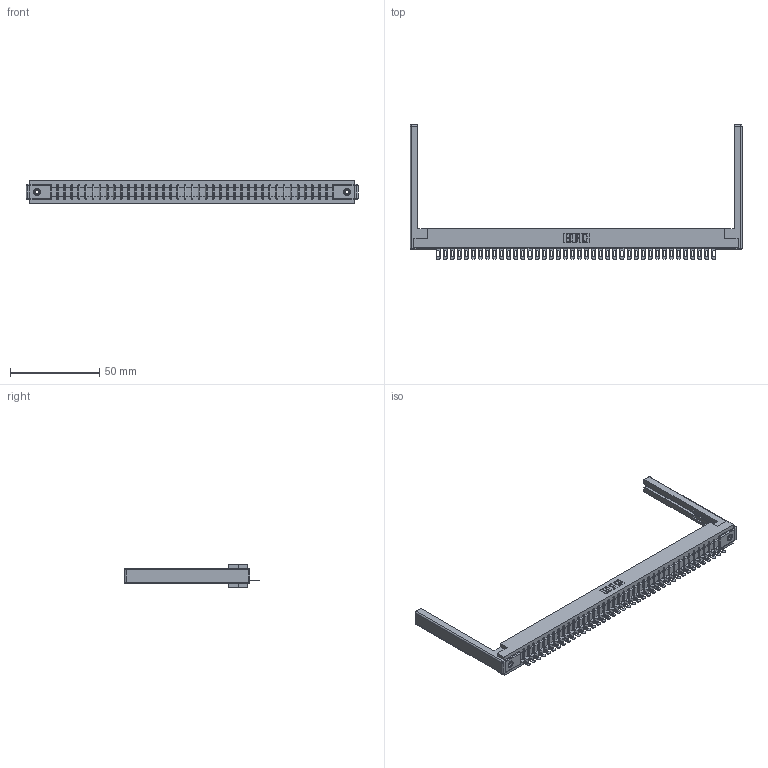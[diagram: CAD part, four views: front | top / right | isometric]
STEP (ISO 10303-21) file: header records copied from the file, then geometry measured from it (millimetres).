
FILE_DESCRIPTION (( 'STEP AP203' ), '1' );
FILE_NAME ('357-040-501-168.STEP', '2019-09-17T08:53:26', ( '' ), ( '' ), 'SwSTEP 2.0', 'SolidWorks 2016', '' );
FILE_SCHEMA (( 'CONFIG_CONTROL_DESIGN' ));
Length unit declared in the file: inch
Products named in the file (5): 307-220-068; 307 Part_.156 Dia Mounting Holes; 345-250-001_345-250-001-102; 357-040-501-168; 307-290-002_501
Assembly tree (45 placements, depth 2):
  357-040-501-168
    307 Part_.156 Dia Mounting Holes
    307-290-002_501  x40
    307-220-068  x2
    345-250-001_345-250-001-102  x2
Bounding box: 185.93 x 75.39 x 12.7 mm (x, y, z)
Volume: 24294.2 mm3; surface area: 29229.7 mm2
Topology: 45 solids, 45 shells, 3353 faces, 10233 edges, 6690 vertices
Faces by surface type: plane 1918, cylinder 1329, sphere 90, cone 12, torus 4
Entity records: 38091 total; most frequent: CARTESIAN_POINT 6389, ORIENTED_EDGE 6368, DIRECTION 6230, EDGE_CURVE 3184, VECTOR 2432, LINE 2432, VERTEX_POINT 2058, AXIS2_PLACEMENT_3D 1899
